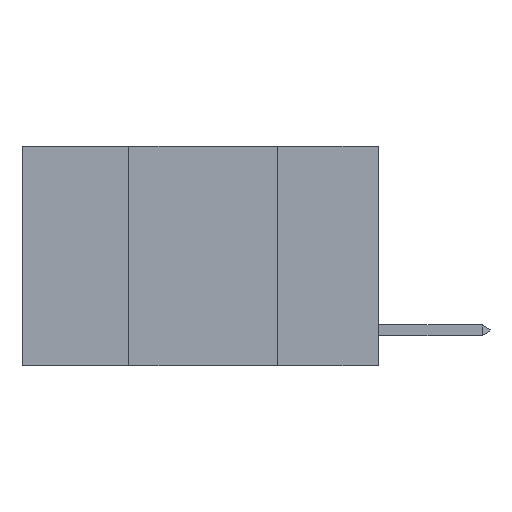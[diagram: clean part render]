
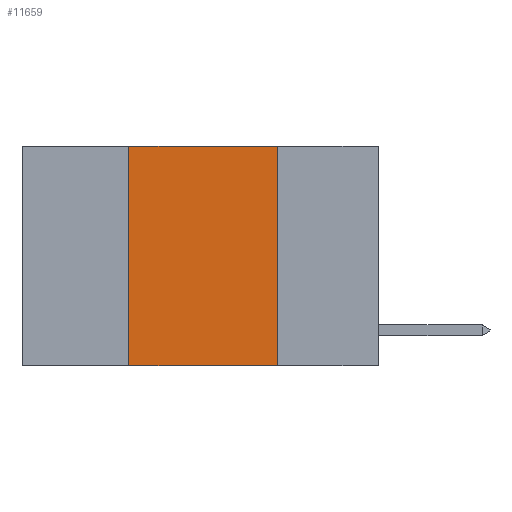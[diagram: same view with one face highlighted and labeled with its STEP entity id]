
A CAD part, left-side view. The second image highlights one B-rep face of the part: STEP entity #11659.
In plain terms, the highlighted planar face has unit normal (-1, 0, 0).
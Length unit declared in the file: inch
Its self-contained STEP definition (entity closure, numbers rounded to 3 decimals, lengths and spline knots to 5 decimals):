
#507 = DIRECTION ( 'NONE',  ( 0., 0., 1. ) ) ;
#545 = CARTESIAN_POINT ( 'NONE',  ( 0., 0.6, 0. ) ) ;
#872 = VECTOR ( 'NONE', #10036, 39.37008 ) ;
#1162 = LINE ( 'NONE', #545, #19426 ) ;
#1729 = VECTOR ( 'NONE', #507, 39.37008 ) ;
#1760 = EDGE_CURVE ( 'NONE', #15129, #20078, #21834, .T. ) ;
#3408 = EDGE_LOOP ( 'NONE', ( #6104, #8660, #18308, #8957 ) ) ;
#3452 = VERTEX_POINT ( 'NONE', #14079 ) ;
#5559 = LINE ( 'NONE', #20676, #872 ) ;
#6104 = ORIENTED_EDGE ( 'NONE', *, *, #21169, .F. ) ;
#6757 = CARTESIAN_POINT ( 'NONE',  ( 0., 0.6, -0.37 ) ) ;
#7898 = VERTEX_POINT ( 'NONE', #22492 ) ;
#7935 = DIRECTION ( 'NONE',  ( 1., 0., 0. ) ) ;
#8660 = ORIENTED_EDGE ( 'NONE', *, *, #20951, .F. ) ;
#8836 = CARTESIAN_POINT ( 'NONE',  ( 0., 0.42, -0.37 ) ) ;
#8957 = ORIENTED_EDGE ( 'NONE', *, *, #1760, .T. ) ;
#9172 = AXIS2_PLACEMENT_3D ( 'NONE', #11227, #7935, #20322 ) ;
#10036 = DIRECTION ( 'NONE',  ( 0., 0., -1. ) ) ;
#10442 = DIRECTION ( 'NONE',  ( 0., -1., 0. ) ) ;
#11227 = CARTESIAN_POINT ( 'NONE',  ( 0., 0.6, 0. ) ) ;
#11659 = ADVANCED_FACE ( 'NONE', ( #21438 ), #18529, .F. ) ;
#14079 = CARTESIAN_POINT ( 'NONE',  ( 0., 0.42, 0. ) ) ;
#15129 = VERTEX_POINT ( 'NONE', #8836 ) ;
#16471 = EDGE_CURVE ( 'NONE', #15129, #3452, #19454, .T. ) ;
#16517 = DIRECTION ( 'NONE',  ( 0., -1., 0. ) ) ;
#17167 = VECTOR ( 'NONE', #10442, 39.37008 ) ;
#17697 = CARTESIAN_POINT ( 'NONE',  ( 0., 0.17, -0.37 ) ) ;
#18308 = ORIENTED_EDGE ( 'NONE', *, *, #16471, .F. ) ;
#18529 = PLANE ( 'NONE',  #9172 ) ;
#19426 = VECTOR ( 'NONE', #16517, 39.37008 ) ;
#19454 = LINE ( 'NONE', #21701, #1729 ) ;
#20078 = VERTEX_POINT ( 'NONE', #17697 ) ;
#20322 = DIRECTION ( 'NONE',  ( 0., 0., -1. ) ) ;
#20676 = CARTESIAN_POINT ( 'NONE',  ( 0., 0.17, 0. ) ) ;
#20951 = EDGE_CURVE ( 'NONE', #3452, #7898, #1162, .T. ) ;
#21169 = EDGE_CURVE ( 'NONE', #7898, #20078, #5559, .T. ) ;
#21438 = FACE_OUTER_BOUND ( 'NONE', #3408, .T. ) ;
#21701 = CARTESIAN_POINT ( 'NONE',  ( 0., 0.42, 0. ) ) ;
#21834 = LINE ( 'NONE', #6757, #17167 ) ;
#22492 = CARTESIAN_POINT ( 'NONE',  ( 0., 0.17, 0. ) ) ;
